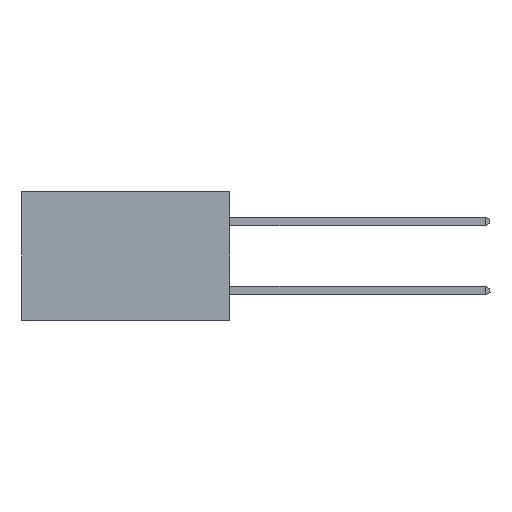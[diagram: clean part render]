
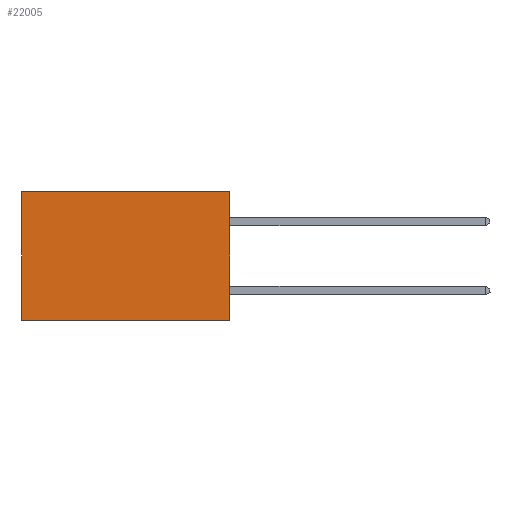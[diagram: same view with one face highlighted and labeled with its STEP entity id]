
A CAD part, left-side view. The second image highlights one B-rep face of the part: STEP entity #22005.
In plain terms, the highlighted planar face has unit normal (-1, 0, 0).
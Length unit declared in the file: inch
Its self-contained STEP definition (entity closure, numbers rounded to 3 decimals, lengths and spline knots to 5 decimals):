
#412 = CARTESIAN_POINT ( 'NONE',  ( 0.298, 0., 0. ) ) ;
#612 = VERTEX_POINT ( 'NONE', #16003 ) ;
#875 = ORIENTED_EDGE ( 'NONE', *, *, #10141, .T. ) ;
#2397 = VECTOR ( 'NONE', #3600, 39.37008 ) ;
#3600 = DIRECTION ( 'NONE',  ( 0., 0., -1. ) ) ;
#6090 = EDGE_CURVE ( 'NONE', #9351, #11895, #14634, .T. ) ;
#7164 = CARTESIAN_POINT ( 'NONE',  ( 0.298, 0., -0.37 ) ) ;
#7707 = VECTOR ( 'NONE', #16899, 39.37008 ) ;
#8511 = ORIENTED_EDGE ( 'NONE', *, *, #8725, .F. ) ;
#8725 = EDGE_CURVE ( 'NONE', #612, #11895, #26812, .T. ) ;
#9351 = VERTEX_POINT ( 'NONE', #26645 ) ;
#9491 = LINE ( 'NONE', #15556, #2397 ) ;
#10141 = EDGE_CURVE ( 'NONE', #15293, #9351, #11020, .T. ) ;
#11020 = LINE ( 'NONE', #20317, #29276 ) ;
#11895 = VERTEX_POINT ( 'NONE', #22418 ) ;
#12885 = DIRECTION ( 'NONE',  ( 1., 0., 0. ) ) ;
#14634 = LINE ( 'NONE', #20580, #27325 ) ;
#15293 = VERTEX_POINT ( 'NONE', #412 ) ;
#15556 = CARTESIAN_POINT ( 'NONE',  ( 0.298, 0., 0. ) ) ;
#16003 = CARTESIAN_POINT ( 'NONE',  ( 0.298, 0., -0.37 ) ) ;
#16899 = DIRECTION ( 'NONE',  ( 0., 1., 0. ) ) ;
#17024 = ORIENTED_EDGE ( 'NONE', *, *, #27292, .F. ) ;
#17833 = FACE_OUTER_BOUND ( 'NONE', #19360, .T. ) ;
#19360 = EDGE_LOOP ( 'NONE', ( #21254, #8511, #17024, #875 ) ) ;
#20317 = CARTESIAN_POINT ( 'NONE',  ( 0.298, 0., 0. ) ) ;
#20577 = DIRECTION ( 'NONE',  ( 0., 0., -1. ) ) ;
#20580 = CARTESIAN_POINT ( 'NONE',  ( 0.298, 0.6, 0. ) ) ;
#21254 = ORIENTED_EDGE ( 'NONE', *, *, #6090, .T. ) ;
#21496 = AXIS2_PLACEMENT_3D ( 'NONE', #27149, #12885, #29499 ) ;
#22005 = ADVANCED_FACE ( 'NONE', ( #17833 ), #29391, .F. ) ;
#22418 = CARTESIAN_POINT ( 'NONE',  ( 0.298, 0.6, -0.37 ) ) ;
#22703 = DIRECTION ( 'NONE',  ( 0., 1., 0. ) ) ;
#26645 = CARTESIAN_POINT ( 'NONE',  ( 0.298, 0.6, 0. ) ) ;
#26812 = LINE ( 'NONE', #7164, #7707 ) ;
#27149 = CARTESIAN_POINT ( 'NONE',  ( 0.298, 0., 0. ) ) ;
#27292 = EDGE_CURVE ( 'NONE', #15293, #612, #9491, .T. ) ;
#27325 = VECTOR ( 'NONE', #20577, 39.37008 ) ;
#29276 = VECTOR ( 'NONE', #22703, 39.37008 ) ;
#29391 = PLANE ( 'NONE',  #21496 ) ;
#29499 = DIRECTION ( 'NONE',  ( 0., 0., -1. ) ) ;
